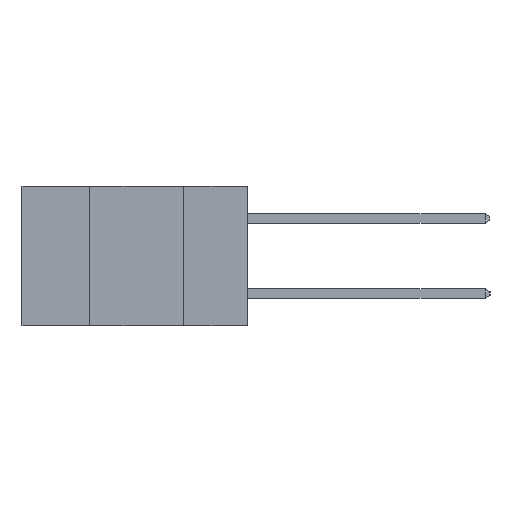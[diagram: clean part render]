
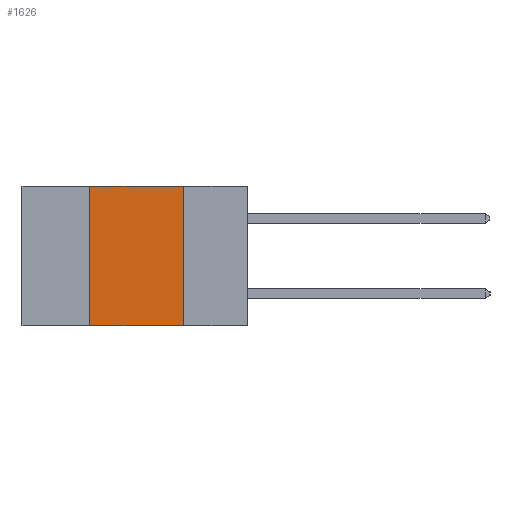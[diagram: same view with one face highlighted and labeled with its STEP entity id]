
A CAD part, left-side view. The second image highlights one B-rep face of the part: STEP entity #1626.
In plain terms, the highlighted planar face has unit normal (-1, 0, 0).
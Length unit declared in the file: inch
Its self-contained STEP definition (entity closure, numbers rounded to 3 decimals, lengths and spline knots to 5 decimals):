
#1 = ORIENTED_EDGE ( 'NONE', *, *, #5879, .F. ) ;
#36 = ORIENTED_EDGE ( 'NONE', *, *, #14248, .F. ) ;
#50 = ORIENTED_EDGE ( 'NONE', *, *, #6818, .T. ) ;
#562 = LINE ( 'NONE', #12631, #6559 ) ;
#783 = VERTEX_POINT ( 'NONE', #5883 ) ;
#968 = LINE ( 'NONE', #1848, #6275 ) ;
#1626 = ADVANCED_FACE ( 'NONE', ( #4477 ), #11975, .F. ) ;
#1848 = CARTESIAN_POINT ( 'NONE',  ( 0., 0.17, -0.37 ) ) ;
#1877 = VERTEX_POINT ( 'NONE', #8879 ) ;
#1992 = DIRECTION ( 'NONE',  ( 0., 0., -1. ) ) ;
#2516 = CARTESIAN_POINT ( 'NONE',  ( 0., 0.17, -0.37 ) ) ;
#2703 = EDGE_LOOP ( 'NONE', ( #4101, #1, #36, #50 ) ) ;
#2802 = CARTESIAN_POINT ( 'NONE',  ( 0., 0.17, 0. ) ) ;
#4101 = ORIENTED_EDGE ( 'NONE', *, *, #12647, .F. ) ;
#4477 = FACE_OUTER_BOUND ( 'NONE', #2703, .T. ) ;
#5879 = EDGE_CURVE ( 'NONE', #1877, #13615, #11172, .T. ) ;
#5883 = CARTESIAN_POINT ( 'NONE',  ( 0., 0.42, -0.37 ) ) ;
#6055 = VECTOR ( 'NONE', #6236, 39.37008 ) ;
#6236 = DIRECTION ( 'NONE',  ( 0., 0., 1. ) ) ;
#6275 = VECTOR ( 'NONE', #1992, 39.37008 ) ;
#6446 = CARTESIAN_POINT ( 'NONE',  ( 0., 0.42, -0.37 ) ) ;
#6559 = VECTOR ( 'NONE', #12614, 39.37008 ) ;
#6818 = EDGE_CURVE ( 'NONE', #783, #11075, #562, .T. ) ;
#8879 = CARTESIAN_POINT ( 'NONE',  ( 0., 0.42, 0. ) ) ;
#8991 = LINE ( 'NONE', #6446, #6055 ) ;
#9387 = DIRECTION ( 'NONE',  ( 0., -1., 0. ) ) ;
#9556 = CARTESIAN_POINT ( 'NONE',  ( 0., 0.6, 0. ) ) ;
#11075 = VERTEX_POINT ( 'NONE', #2516 ) ;
#11172 = LINE ( 'NONE', #9556, #13718 ) ;
#11854 = DIRECTION ( 'NONE',  ( 0., 0., -1. ) ) ;
#11903 = DIRECTION ( 'NONE',  ( 1., 0., 0. ) ) ;
#11975 = PLANE ( 'NONE',  #13875 ) ;
#11990 = CARTESIAN_POINT ( 'NONE',  ( 0., 0.6, 0. ) ) ;
#12614 = DIRECTION ( 'NONE',  ( 0., -1., 0. ) ) ;
#12631 = CARTESIAN_POINT ( 'NONE',  ( 0., 0.6, -0.37 ) ) ;
#12647 = EDGE_CURVE ( 'NONE', #13615, #11075, #968, .T. ) ;
#13615 = VERTEX_POINT ( 'NONE', #2802 ) ;
#13718 = VECTOR ( 'NONE', #9387, 39.37008 ) ;
#13875 = AXIS2_PLACEMENT_3D ( 'NONE', #11990, #11903, #11854 ) ;
#14248 = EDGE_CURVE ( 'NONE', #783, #1877, #8991, .T. ) ;
